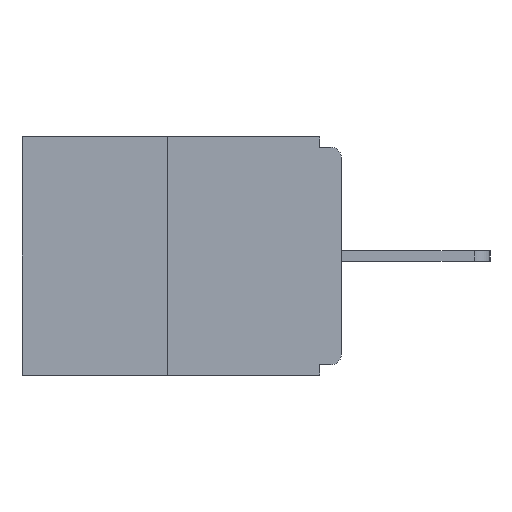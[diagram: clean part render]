
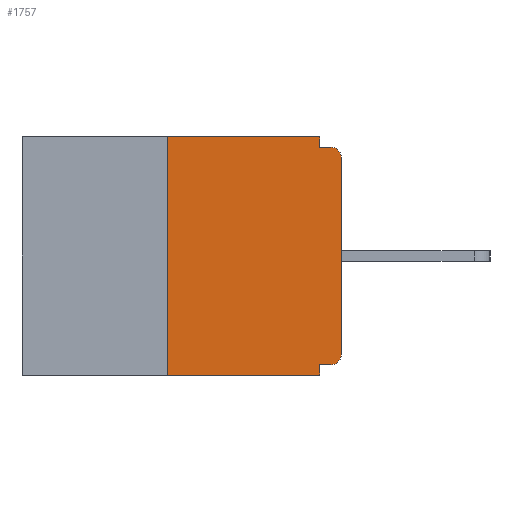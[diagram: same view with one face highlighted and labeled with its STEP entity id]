
A CAD part, left-side view. The second image highlights one B-rep face of the part: STEP entity #1757.
In plain terms, the highlighted planar face has unit normal (-1, 0, 0).
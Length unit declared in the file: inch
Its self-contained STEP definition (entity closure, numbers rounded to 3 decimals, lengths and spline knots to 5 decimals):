
#74 = VERTEX_POINT ( 'NONE', #6230 ) ;
#649 = CARTESIAN_POINT ( 'NONE',  ( 0., 0.031, -0.015 ) ) ;
#891 = CARTESIAN_POINT ( 'NONE',  ( 0., 0., 0. ) ) ;
#906 = LINE ( 'NONE', #13275, #7594 ) ;
#942 = VERTEX_POINT ( 'NONE', #3855 ) ;
#1269 = LINE ( 'NONE', #5852, #8969 ) ;
#1283 = CARTESIAN_POINT ( 'NONE',  ( 0., 0.031, 0. ) ) ;
#1314 = DIRECTION ( 'NONE',  ( 0., 0., -1. ) ) ;
#1337 = ORIENTED_EDGE ( 'NONE', *, *, #13586, .F. ) ;
#1757 = ADVANCED_FACE ( 'NONE', ( #9722 ), #7423, .F. ) ;
#1882 = ORIENTED_EDGE ( 'NONE', *, *, #9136, .T. ) ;
#1883 = VERTEX_POINT ( 'NONE', #6472 ) ;
#1907 = VERTEX_POINT ( 'NONE', #12150 ) ;
#2037 = DIRECTION ( 'NONE',  ( 0., 0., -1. ) ) ;
#2172 = CARTESIAN_POINT ( 'NONE',  ( 0., 0.46, 0. ) ) ;
#2295 = EDGE_CURVE ( 'NONE', #74, #2570, #11022, .T. ) ;
#2570 = VERTEX_POINT ( 'NONE', #8423 ) ;
#2716 = CARTESIAN_POINT ( 'NONE',  ( 0., 0., -0.03 ) ) ;
#3215 = EDGE_CURVE ( 'NONE', #1883, #1907, #1269, .T. ) ;
#3417 = VERTEX_POINT ( 'NONE', #649 ) ;
#3423 = DIRECTION ( 'NONE',  ( 0., -1., 0. ) ) ;
#3478 = DIRECTION ( 'NONE',  ( 0., 1., 0. ) ) ;
#3855 = CARTESIAN_POINT ( 'NONE',  ( 0., 0.25, 0. ) ) ;
#4082 = CARTESIAN_POINT ( 'NONE',  ( 0., 0.46, 0. ) ) ;
#4300 = AXIS2_PLACEMENT_3D ( 'NONE', #8302, #12831, #12746 ) ;
#4659 = VERTEX_POINT ( 'NONE', #11783 ) ;
#5419 = DIRECTION ( 'NONE',  ( 0., 0., 1. ) ) ;
#5852 = CARTESIAN_POINT ( 'NONE',  ( 0., 0., -0.328 ) ) ;
#5941 = VECTOR ( 'NONE', #12137, 39.37008 ) ;
#6209 = EDGE_CURVE ( 'NONE', #942, #4659, #12315, .T. ) ;
#6230 = CARTESIAN_POINT ( 'NONE',  ( 0., 0.25, -0.343 ) ) ;
#6472 = CARTESIAN_POINT ( 'NONE',  ( 0., 0.015, -0.328 ) ) ;
#6514 = CARTESIAN_POINT ( 'NONE',  ( 0., 0.015, -0.015 ) ) ;
#6711 = DIRECTION ( 'NONE',  ( 0., -1., 0. ) ) ;
#6755 = LINE ( 'NONE', #891, #7347 ) ;
#6959 = CARTESIAN_POINT ( 'NONE',  ( 0., 0.015, -0.03 ) ) ;
#7054 = AXIS2_PLACEMENT_3D ( 'NONE', #4082, #9794, #8390 ) ;
#7068 = AXIS2_PLACEMENT_3D ( 'NONE', #6959, #11454, #1314 ) ;
#7146 = CIRCLE ( 'NONE', #4300, 0.015 ) ;
#7301 = VECTOR ( 'NONE', #2037, 39.37008 ) ;
#7347 = VECTOR ( 'NONE', #5419, 39.37008 ) ;
#7423 = PLANE ( 'NONE',  #7054 ) ;
#7594 = VECTOR ( 'NONE', #3423, 39.37008 ) ;
#7902 = CARTESIAN_POINT ( 'NONE',  ( 0., 0.031, -0.343 ) ) ;
#8017 = CARTESIAN_POINT ( 'NONE',  ( 0., 0.25, 0. ) ) ;
#8052 = EDGE_CURVE ( 'NONE', #1883, #10372, #7146, .T. ) ;
#8062 = VECTOR ( 'NONE', #8167, 39.37008 ) ;
#8167 = DIRECTION ( 'NONE',  ( 0., 0., -1. ) ) ;
#8176 = ORIENTED_EDGE ( 'NONE', *, *, #9366, .F. ) ;
#8302 = CARTESIAN_POINT ( 'NONE',  ( 0., 0.015, -0.313 ) ) ;
#8390 = DIRECTION ( 'NONE',  ( 0., 0., -1. ) ) ;
#8423 = CARTESIAN_POINT ( 'NONE',  ( 0., 0.031, -0.343 ) ) ;
#8552 = VERTEX_POINT ( 'NONE', #6514 ) ;
#8597 = ORIENTED_EDGE ( 'NONE', *, *, #2295, .T. ) ;
#8969 = VECTOR ( 'NONE', #3478, 39.37008 ) ;
#9034 = VECTOR ( 'NONE', #12534, 39.37008 ) ;
#9110 = VERTEX_POINT ( 'NONE', #2716 ) ;
#9136 = EDGE_CURVE ( 'NONE', #9110, #8552, #10832, .T. ) ;
#9366 = EDGE_CURVE ( 'NONE', #1907, #2570, #13513, .T. ) ;
#9551 = CARTESIAN_POINT ( 'NONE',  ( 0., 0., -0.313 ) ) ;
#9722 = FACE_OUTER_BOUND ( 'NONE', #12435, .T. ) ;
#9794 = DIRECTION ( 'NONE',  ( 1., 0., 0. ) ) ;
#10372 = VERTEX_POINT ( 'NONE', #9551 ) ;
#10378 = LINE ( 'NONE', #8017, #9034 ) ;
#10443 = ORIENTED_EDGE ( 'NONE', *, *, #13775, .F. ) ;
#10832 = CIRCLE ( 'NONE', #7068, 0.015 ) ;
#10952 = CARTESIAN_POINT ( 'NONE',  ( 0., 0.46, -0.343 ) ) ;
#11022 = LINE ( 'NONE', #10952, #5941 ) ;
#11319 = EDGE_CURVE ( 'NONE', #4659, #3417, #13857, .T. ) ;
#11454 = DIRECTION ( 'NONE',  ( -1., 0., 0. ) ) ;
#11783 = CARTESIAN_POINT ( 'NONE',  ( 0., 0.031, 0. ) ) ;
#11828 = ORIENTED_EDGE ( 'NONE', *, *, #11319, .F. ) ;
#12137 = DIRECTION ( 'NONE',  ( 0., -1., 0. ) ) ;
#12150 = CARTESIAN_POINT ( 'NONE',  ( 0., 0.031, -0.328 ) ) ;
#12315 = LINE ( 'NONE', #2172, #14175 ) ;
#12435 = EDGE_LOOP ( 'NONE', ( #13465, #10443, #8597, #8176, #12567, #12910, #12448, #1882, #1337, #11828 ) ) ;
#12448 = ORIENTED_EDGE ( 'NONE', *, *, #12938, .T. ) ;
#12534 = DIRECTION ( 'NONE',  ( 0., 0., 1. ) ) ;
#12567 = ORIENTED_EDGE ( 'NONE', *, *, #3215, .F. ) ;
#12746 = DIRECTION ( 'NONE',  ( 0., 0., -1. ) ) ;
#12831 = DIRECTION ( 'NONE',  ( -1., 0., 0. ) ) ;
#12910 = ORIENTED_EDGE ( 'NONE', *, *, #8052, .T. ) ;
#12938 = EDGE_CURVE ( 'NONE', #10372, #9110, #6755, .T. ) ;
#13275 = CARTESIAN_POINT ( 'NONE',  ( 0., 0., -0.015 ) ) ;
#13465 = ORIENTED_EDGE ( 'NONE', *, *, #6209, .F. ) ;
#13513 = LINE ( 'NONE', #7902, #7301 ) ;
#13586 = EDGE_CURVE ( 'NONE', #3417, #8552, #906, .T. ) ;
#13775 = EDGE_CURVE ( 'NONE', #74, #942, #10378, .T. ) ;
#13857 = LINE ( 'NONE', #1283, #8062 ) ;
#14175 = VECTOR ( 'NONE', #6711, 39.37008 ) ;
